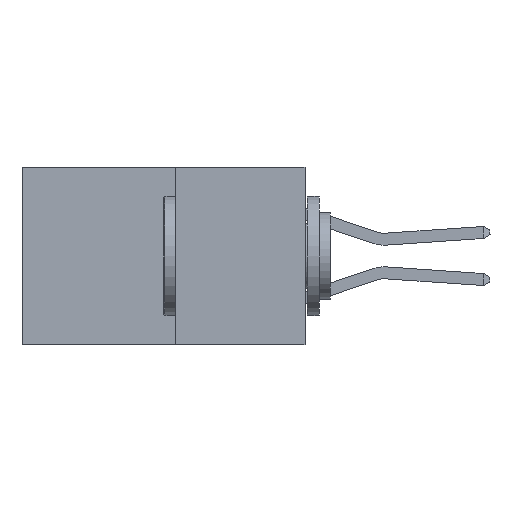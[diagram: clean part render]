
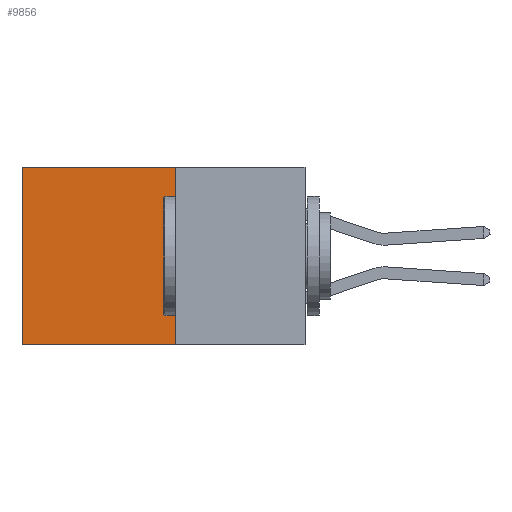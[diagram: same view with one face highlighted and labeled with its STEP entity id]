
A CAD part, left-side view. The second image highlights one B-rep face of the part: STEP entity #9856.
In plain terms, the highlighted planar face has unit normal (-1, 0, 0).
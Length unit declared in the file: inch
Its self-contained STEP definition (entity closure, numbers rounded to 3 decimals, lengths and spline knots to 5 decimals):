
#155 = CARTESIAN_POINT ( 'NONE',  ( 0.277, 0.59, -0.37 ) ) ;
#340 = LINE ( 'NONE', #5102, #13925 ) ;
#1336 = EDGE_CURVE ( 'NONE', #11752, #16311, #3928, .T. ) ;
#1749 = CARTESIAN_POINT ( 'NONE',  ( 0.277, 0.59, -0.37 ) ) ;
#2071 = CARTESIAN_POINT ( 'NONE',  ( 0.277, 0.27, 0. ) ) ;
#2502 = EDGE_CURVE ( 'NONE', #10274, #15056, #4109, .T. ) ;
#3754 = ORIENTED_EDGE ( 'NONE', *, *, #14485, .T. ) ;
#3787 = ORIENTED_EDGE ( 'NONE', *, *, #2502, .F. ) ;
#3887 = ORIENTED_EDGE ( 'NONE', *, *, #10189, .F. ) ;
#3928 = LINE ( 'NONE', #2071, #13907 ) ;
#4109 = LINE ( 'NONE', #9563, #8763 ) ;
#4129 = CARTESIAN_POINT ( 'NONE',  ( 0.277, 0.27, 0. ) ) ;
#4191 = PLANE ( 'NONE',  #15104 ) ;
#4220 = ORIENTED_EDGE ( 'NONE', *, *, #1336, .T. ) ;
#4324 = CARTESIAN_POINT ( 'NONE',  ( 0.277, 0.59, 0. ) ) ;
#4666 = VECTOR ( 'NONE', #9654, 39.37008 ) ;
#5102 = CARTESIAN_POINT ( 'NONE',  ( 0.277, 0.27, -0.37 ) ) ;
#6204 = DIRECTION ( 'NONE',  ( 0., 1., 0. ) ) ;
#6515 = CARTESIAN_POINT ( 'NONE',  ( 0.277, 0.27, -0.37 ) ) ;
#6573 = FACE_OUTER_BOUND ( 'NONE', #10988, .T. ) ;
#6751 = CARTESIAN_POINT ( 'NONE',  ( 0.277, 0.27, -0.37 ) ) ;
#7551 = DIRECTION ( 'NONE',  ( 0., 1., 0. ) ) ;
#8067 = DIRECTION ( 'NONE',  ( 0., 0., -1. ) ) ;
#8763 = VECTOR ( 'NONE', #7551, 39.37008 ) ;
#9563 = CARTESIAN_POINT ( 'NONE',  ( 0.277, 0.27, -0.37 ) ) ;
#9654 = DIRECTION ( 'NONE',  ( 0., 0., -1. ) ) ;
#9856 = ADVANCED_FACE ( 'NONE', ( #6573 ), #4191, .F. ) ;
#10189 = EDGE_CURVE ( 'NONE', #11752, #10274, #340, .T. ) ;
#10274 = VERTEX_POINT ( 'NONE', #6515 ) ;
#10988 = EDGE_LOOP ( 'NONE', ( #3754, #3787, #3887, #4220 ) ) ;
#11591 = LINE ( 'NONE', #1749, #4666 ) ;
#11752 = VERTEX_POINT ( 'NONE', #4129 ) ;
#13907 = VECTOR ( 'NONE', #6204, 39.37008 ) ;
#13925 = VECTOR ( 'NONE', #15412, 39.37008 ) ;
#14485 = EDGE_CURVE ( 'NONE', #16311, #15056, #11591, .T. ) ;
#15056 = VERTEX_POINT ( 'NONE', #155 ) ;
#15104 = AXIS2_PLACEMENT_3D ( 'NONE', #6751, #15793, #8067 ) ;
#15412 = DIRECTION ( 'NONE',  ( 0., 0., -1. ) ) ;
#15793 = DIRECTION ( 'NONE',  ( 1., 0., 0. ) ) ;
#16311 = VERTEX_POINT ( 'NONE', #4324 ) ;
